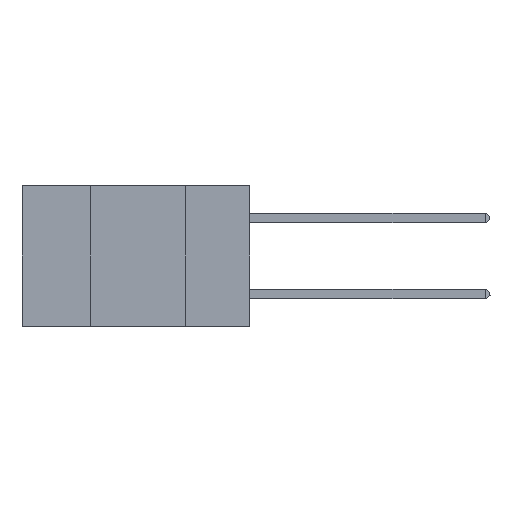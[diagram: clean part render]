
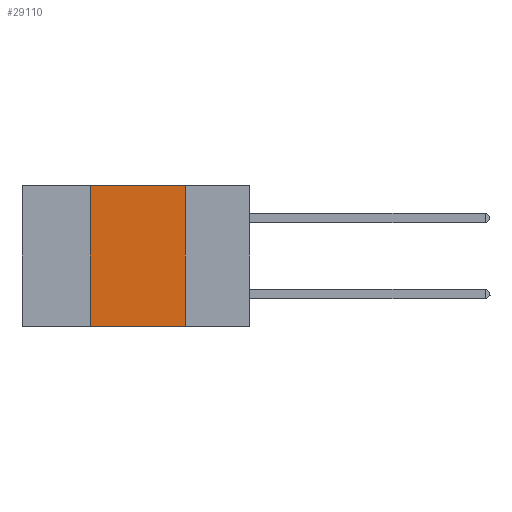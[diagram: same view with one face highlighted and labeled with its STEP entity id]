
A CAD part, left-side view. The second image highlights one B-rep face of the part: STEP entity #29110.
In plain terms, the highlighted planar face has unit normal (-1, 0, 0).
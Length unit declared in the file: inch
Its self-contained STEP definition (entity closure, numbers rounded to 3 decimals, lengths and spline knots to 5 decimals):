
#373 = VERTEX_POINT ( 'NONE', #27062 ) ;
#1243 = DIRECTION ( 'NONE',  ( 0., -1., 0. ) ) ;
#1854 = ORIENTED_EDGE ( 'NONE', *, *, #14375, .F. ) ;
#2382 = ORIENTED_EDGE ( 'NONE', *, *, #12945, .T. ) ;
#2422 = EDGE_LOOP ( 'NONE', ( #12025, #1854, #22061, #2382 ) ) ;
#4381 = CARTESIAN_POINT ( 'NONE',  ( 0., 0.17, 0. ) ) ;
#4928 = FACE_OUTER_BOUND ( 'NONE', #2422, .T. ) ;
#5364 = LINE ( 'NONE', #4381, #9866 ) ;
#7914 = CARTESIAN_POINT ( 'NONE',  ( 0., 0.42, 0. ) ) ;
#8721 = CARTESIAN_POINT ( 'NONE',  ( 0., 0.6, -0.37 ) ) ;
#9076 = VECTOR ( 'NONE', #26935, 39.37008 ) ;
#9110 = CARTESIAN_POINT ( 'NONE',  ( 0., 0.6, 0. ) ) ;
#9866 = VECTOR ( 'NONE', #20849, 39.37008 ) ;
#11052 = VERTEX_POINT ( 'NONE', #25714 ) ;
#12025 = ORIENTED_EDGE ( 'NONE', *, *, #14515, .F. ) ;
#12682 = CARTESIAN_POINT ( 'NONE',  ( 0., 0.42, 0. ) ) ;
#12945 = EDGE_CURVE ( 'NONE', #11052, #17460, #20155, .T. ) ;
#13708 = PLANE ( 'NONE',  #21275 ) ;
#13830 = DIRECTION ( 'NONE',  ( 0., -1., 0. ) ) ;
#14375 = EDGE_CURVE ( 'NONE', #28778, #373, #15580, .T. ) ;
#14404 = VECTOR ( 'NONE', #1243, 39.37008 ) ;
#14515 = EDGE_CURVE ( 'NONE', #373, #17460, #5364, .T. ) ;
#15580 = LINE ( 'NONE', #15688, #14404 ) ;
#15688 = CARTESIAN_POINT ( 'NONE',  ( 0., 0.6, 0. ) ) ;
#17460 = VERTEX_POINT ( 'NONE', #24586 ) ;
#18472 = DIRECTION ( 'NONE',  ( 0., 0., -1. ) ) ;
#20155 = LINE ( 'NONE', #8721, #27300 ) ;
#20849 = DIRECTION ( 'NONE',  ( 0., 0., -1. ) ) ;
#21127 = DIRECTION ( 'NONE',  ( 1., 0., 0. ) ) ;
#21275 = AXIS2_PLACEMENT_3D ( 'NONE', #9110, #21127, #18472 ) ;
#22061 = ORIENTED_EDGE ( 'NONE', *, *, #23750, .F. ) ;
#23750 = EDGE_CURVE ( 'NONE', #11052, #28778, #29016, .T. ) ;
#24586 = CARTESIAN_POINT ( 'NONE',  ( 0., 0.17, -0.37 ) ) ;
#25714 = CARTESIAN_POINT ( 'NONE',  ( 0., 0.42, -0.37 ) ) ;
#26935 = DIRECTION ( 'NONE',  ( 0., 0., 1. ) ) ;
#27062 = CARTESIAN_POINT ( 'NONE',  ( 0., 0.17, 0. ) ) ;
#27300 = VECTOR ( 'NONE', #13830, 39.37008 ) ;
#28778 = VERTEX_POINT ( 'NONE', #12682 ) ;
#29016 = LINE ( 'NONE', #7914, #9076 ) ;
#29110 = ADVANCED_FACE ( 'NONE', ( #4928 ), #13708, .F. ) ;
